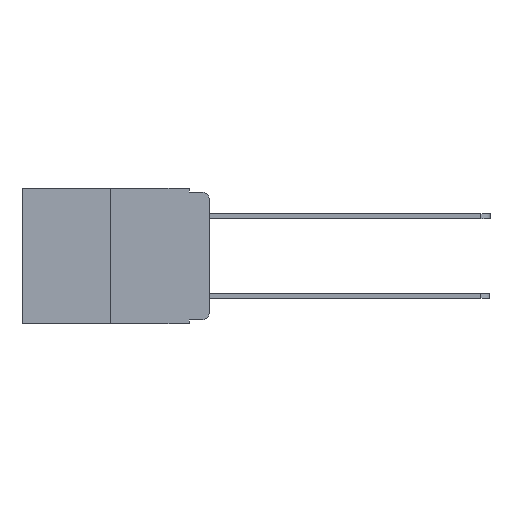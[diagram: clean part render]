
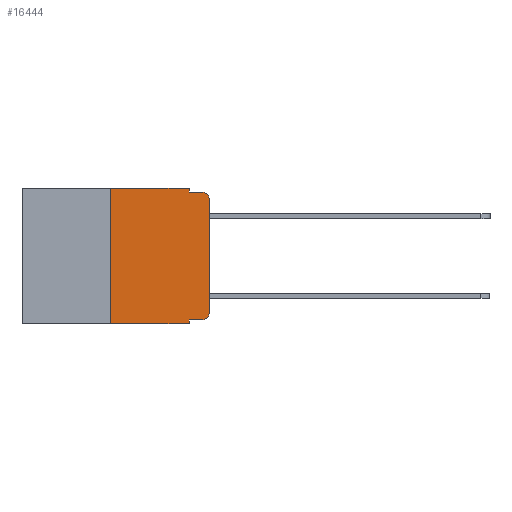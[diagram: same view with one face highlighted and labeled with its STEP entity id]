
A CAD part, left-side view. The second image highlights one B-rep face of the part: STEP entity #16444.
In plain terms, the highlighted planar face has unit normal (-1, 0, 0).
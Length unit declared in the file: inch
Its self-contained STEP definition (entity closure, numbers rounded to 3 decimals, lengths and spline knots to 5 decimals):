
#231 = LINE ( 'NONE', #3419, #13923 ) ;
#721 = VERTEX_POINT ( 'NONE', #14453 ) ;
#740 = CARTESIAN_POINT ( 'NONE',  ( 0., 0.25, 0. ) ) ;
#859 = EDGE_CURVE ( 'NONE', #12466, #14864, #15109, .T. ) ;
#979 = EDGE_LOOP ( 'NONE', ( #4969, #2704, #3925, #11343, #7192, #11535, #10602, #12480, #3752, #10235 ) ) ;
#1159 = EDGE_CURVE ( 'NONE', #16121, #11172, #6693, .T. ) ;
#1282 = EDGE_CURVE ( 'NONE', #4028, #721, #9760, .T. ) ;
#1460 = DIRECTION ( 'NONE',  ( 0., -1., 0. ) ) ;
#1557 = EDGE_CURVE ( 'NONE', #12131, #11172, #231, .T. ) ;
#1615 = LINE ( 'NONE', #5875, #14588 ) ;
#1668 = DIRECTION ( 'NONE',  ( 0., 0., -1. ) ) ;
#1764 = VECTOR ( 'NONE', #5283, 39.37008 ) ;
#2169 = CIRCLE ( 'NONE', #12744, 0.02 ) ;
#2589 = EDGE_CURVE ( 'NONE', #5386, #13468, #2169, .T. ) ;
#2607 = AXIS2_PLACEMENT_3D ( 'NONE', #11728, #9358, #1668 ) ;
#2693 = AXIS2_PLACEMENT_3D ( 'NONE', #11886, #4470, #13089 ) ;
#2704 = ORIENTED_EDGE ( 'NONE', *, *, #1159, .T. ) ;
#3176 = EDGE_CURVE ( 'NONE', #9636, #12466, #6838, .T. ) ;
#3419 = CARTESIAN_POINT ( 'NONE',  ( 0., 0.051, -0.01 ) ) ;
#3482 = CARTESIAN_POINT ( 'NONE',  ( 0., 0.051, -0.01 ) ) ;
#3752 = ORIENTED_EDGE ( 'NONE', *, *, #15963, .T. ) ;
#3915 = DIRECTION ( 'NONE',  ( 0., -1., 0. ) ) ;
#3925 = ORIENTED_EDGE ( 'NONE', *, *, #1557, .F. ) ;
#4028 = VERTEX_POINT ( 'NONE', #15857 ) ;
#4114 = CARTESIAN_POINT ( 'NONE',  ( 0., 0.473, -0.343 ) ) ;
#4245 = CARTESIAN_POINT ( 'NONE',  ( 0., 0.25, -0.343 ) ) ;
#4470 = DIRECTION ( 'NONE',  ( -1., 0., 0. ) ) ;
#4652 = VECTOR ( 'NONE', #1460, 39.37008 ) ;
#4768 = DIRECTION ( 'NONE',  ( 0., 0., 1. ) ) ;
#4907 = DIRECTION ( 'NONE',  ( 0., 0., 1. ) ) ;
#4969 = ORIENTED_EDGE ( 'NONE', *, *, #16639, .T. ) ;
#4973 = CARTESIAN_POINT ( 'NONE',  ( 0., 0.051, 0. ) ) ;
#5283 = DIRECTION ( 'NONE',  ( 0., 0., -1. ) ) ;
#5386 = VERTEX_POINT ( 'NONE', #8764 ) ;
#5875 = CARTESIAN_POINT ( 'NONE',  ( 0., 0.051, -0.333 ) ) ;
#6305 = EDGE_CURVE ( 'NONE', #9636, #721, #8021, .T. ) ;
#6486 = VECTOR ( 'NONE', #12337, 39.37008 ) ;
#6693 = CIRCLE ( 'NONE', #2693, 0.02 ) ;
#6838 = LINE ( 'NONE', #740, #12523 ) ;
#7083 = CARTESIAN_POINT ( 'NONE',  ( 0., 0.473, 0. ) ) ;
#7192 = ORIENTED_EDGE ( 'NONE', *, *, #859, .F. ) ;
#7853 = CARTESIAN_POINT ( 'NONE',  ( 0., 0.02, -0.313 ) ) ;
#8021 = LINE ( 'NONE', #4114, #4652 ) ;
#8143 = PLANE ( 'NONE',  #2607 ) ;
#8382 = DIRECTION ( 'NONE',  ( 0., -1., 0. ) ) ;
#8764 = CARTESIAN_POINT ( 'NONE',  ( 0., 0.02, -0.333 ) ) ;
#9091 = DIRECTION ( 'NONE',  ( 0., 0., -1. ) ) ;
#9256 = CARTESIAN_POINT ( 'NONE',  ( 0., 0.051, 0. ) ) ;
#9358 = DIRECTION ( 'NONE',  ( 1., 0., 0. ) ) ;
#9480 = CARTESIAN_POINT ( 'NONE',  ( 0., 0.02, -0.01 ) ) ;
#9609 = VECTOR ( 'NONE', #4768, 39.37008 ) ;
#9636 = VERTEX_POINT ( 'NONE', #4245 ) ;
#9760 = LINE ( 'NONE', #4973, #6486 ) ;
#10235 = ORIENTED_EDGE ( 'NONE', *, *, #2589, .T. ) ;
#10602 = ORIENTED_EDGE ( 'NONE', *, *, #6305, .T. ) ;
#11143 = CARTESIAN_POINT ( 'NONE',  ( 0., 0., -0.03 ) ) ;
#11172 = VERTEX_POINT ( 'NONE', #9480 ) ;
#11188 = CARTESIAN_POINT ( 'NONE',  ( 0., 0., -0.313 ) ) ;
#11343 = ORIENTED_EDGE ( 'NONE', *, *, #13153, .F. ) ;
#11424 = CARTESIAN_POINT ( 'NONE',  ( 0., 0.25, 0. ) ) ;
#11535 = ORIENTED_EDGE ( 'NONE', *, *, #3176, .F. ) ;
#11728 = CARTESIAN_POINT ( 'NONE',  ( 0., 0.473, 0. ) ) ;
#11873 = VECTOR ( 'NONE', #3915, 39.37008 ) ;
#11886 = CARTESIAN_POINT ( 'NONE',  ( 0., 0.02, -0.03 ) ) ;
#12129 = DIRECTION ( 'NONE',  ( 0., -1., 0. ) ) ;
#12131 = VERTEX_POINT ( 'NONE', #3482 ) ;
#12337 = DIRECTION ( 'NONE',  ( 0., 0., -1. ) ) ;
#12466 = VERTEX_POINT ( 'NONE', #11424 ) ;
#12480 = ORIENTED_EDGE ( 'NONE', *, *, #1282, .F. ) ;
#12523 = VECTOR ( 'NONE', #4907, 39.37008 ) ;
#12609 = FACE_OUTER_BOUND ( 'NONE', #979, .T. ) ;
#12744 = AXIS2_PLACEMENT_3D ( 'NONE', #7853, #16398, #9091 ) ;
#13089 = DIRECTION ( 'NONE',  ( 0., 0., -1. ) ) ;
#13153 = EDGE_CURVE ( 'NONE', #14864, #12131, #15074, .T. ) ;
#13468 = VERTEX_POINT ( 'NONE', #11188 ) ;
#13923 = VECTOR ( 'NONE', #12129, 39.37008 ) ;
#14453 = CARTESIAN_POINT ( 'NONE',  ( 0., 0.051, -0.343 ) ) ;
#14567 = CARTESIAN_POINT ( 'NONE',  ( 0., 0., 0. ) ) ;
#14588 = VECTOR ( 'NONE', #8382, 39.37008 ) ;
#14864 = VERTEX_POINT ( 'NONE', #9256 ) ;
#15074 = LINE ( 'NONE', #15089, #1764 ) ;
#15089 = CARTESIAN_POINT ( 'NONE',  ( 0., 0.051, 0. ) ) ;
#15109 = LINE ( 'NONE', #7083, #11873 ) ;
#15857 = CARTESIAN_POINT ( 'NONE',  ( 0., 0.051, -0.333 ) ) ;
#15963 = EDGE_CURVE ( 'NONE', #4028, #5386, #1615, .T. ) ;
#16112 = LINE ( 'NONE', #14567, #9609 ) ;
#16121 = VERTEX_POINT ( 'NONE', #11143 ) ;
#16398 = DIRECTION ( 'NONE',  ( -1., 0., 0. ) ) ;
#16444 = ADVANCED_FACE ( 'NONE', ( #12609 ), #8143, .F. ) ;
#16639 = EDGE_CURVE ( 'NONE', #13468, #16121, #16112, .T. ) ;
